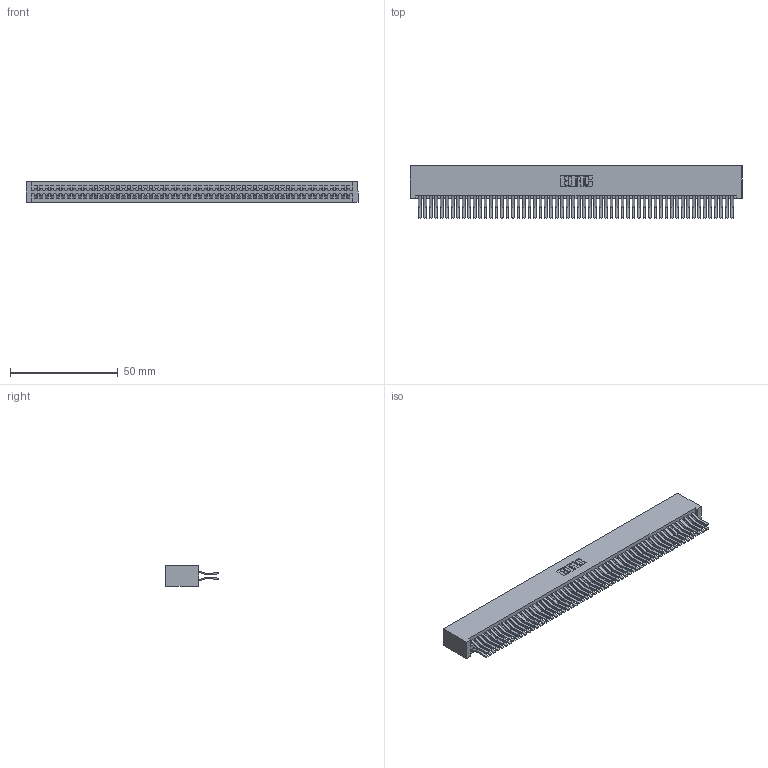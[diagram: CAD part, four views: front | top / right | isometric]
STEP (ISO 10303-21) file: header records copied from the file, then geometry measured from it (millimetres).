
FILE_DESCRIPTION (( 'STEP AP203' ), '1' );
FILE_NAME ('395-116-560-201.STEP', '2018-12-02T03:50:24', ( '' ), ( '' ), 'SwSTEP 2.0', 'SolidWorks 2016', '' );
FILE_SCHEMA (( 'CONFIG_CONTROL_DESIGN' ));
Length unit declared in the file: inch
Products named in the file (3): 345-292-001_560 Tail; 345 Part_No Mounting Lugs; 395-116-560-201
Assembly tree (117 placements, depth 2):
  395-116-560-201
    345 Part_No Mounting Lugs
    345-292-001_560 Tail  x116
Bounding box: 153.92 x 24.45 x 9.4 mm (x, y, z)
Volume: 16477.1 mm3; surface area: 26924.6 mm2
Topology: 117 solids, 117 shells, 6150 faces, 18297 edges, 12042 vertices
Faces by surface type: plane 3904, cylinder 2246
Entity records: 43165 total; most frequent: CARTESIAN_POINT 7220, ORIENTED_EDGE 7154, DIRECTION 6345, EDGE_CURVE 3577, VECTOR 3217, LINE 3217, VERTEX_POINT 2382, AXIS2_PLACEMENT_3D 1564
